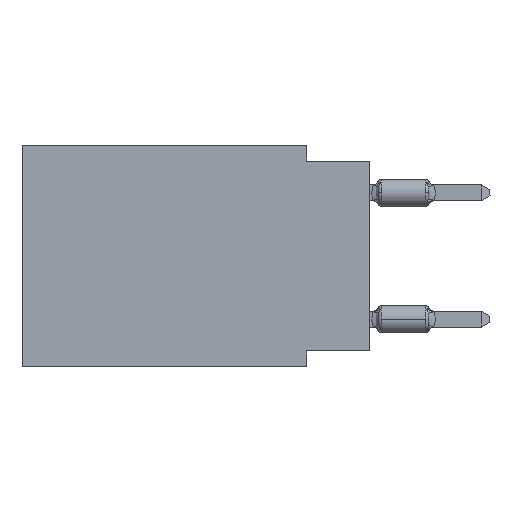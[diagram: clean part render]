
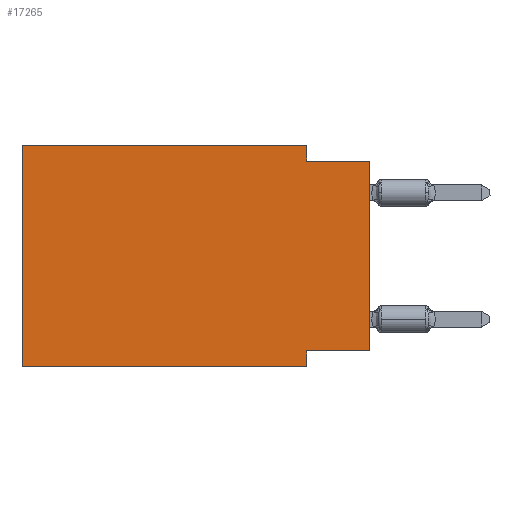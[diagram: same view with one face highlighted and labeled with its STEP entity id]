
A CAD part, left-side view. The second image highlights one B-rep face of the part: STEP entity #17265.
In plain terms, the highlighted planar face has unit normal (-1, 0, 0).
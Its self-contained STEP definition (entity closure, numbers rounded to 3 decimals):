
#519 = VERTEX_POINT ( 'NONE', #16517 ) ;
#940 = CARTESIAN_POINT ( 'NONE',  ( 0., 0., -0.635 ) ) ;
#1024 = LINE ( 'NONE', #8169, #1811 ) ;
#1096 = VERTEX_POINT ( 'NONE', #8989 ) ;
#1276 = VERTEX_POINT ( 'NONE', #13094 ) ;
#1332 = ORIENTED_EDGE ( 'NONE', *, *, #19990, .T. ) ;
#1726 = VERTEX_POINT ( 'NONE', #18130 ) ;
#1811 = VECTOR ( 'NONE', #10003, 1000. ) ;
#2099 = DIRECTION ( 'NONE',  ( 1., 0., 0. ) ) ;
#3362 = LINE ( 'NONE', #19885, #15245 ) ;
#3372 = ORIENTED_EDGE ( 'NONE', *, *, #19219, .F. ) ;
#3564 = ORIENTED_EDGE ( 'NONE', *, *, #18796, .F. ) ;
#4225 = CARTESIAN_POINT ( 'NONE',  ( 0., 0., 0. ) ) ;
#4650 = EDGE_CURVE ( 'NONE', #1726, #1096, #1024, .T. ) ;
#5056 = CARTESIAN_POINT ( 'NONE',  ( 0., 13.97, 0. ) ) ;
#5437 = DIRECTION ( 'NONE',  ( 0., 0., -1. ) ) ;
#5679 = VECTOR ( 'NONE', #12805, 1000. ) ;
#6331 = LINE ( 'NONE', #5056, #10864 ) ;
#6379 = VERTEX_POINT ( 'NONE', #21071 ) ;
#6448 = DIRECTION ( 'NONE',  ( 0., 1., 0. ) ) ;
#6913 = ORIENTED_EDGE ( 'NONE', *, *, #20837, .F. ) ;
#7190 = VECTOR ( 'NONE', #6448, 1000. ) ;
#7294 = PLANE ( 'NONE',  #21196 ) ;
#7486 = ORIENTED_EDGE ( 'NONE', *, *, #20045, .T. ) ;
#7638 = EDGE_CURVE ( 'NONE', #1096, #1276, #22091, .T. ) ;
#7876 = VECTOR ( 'NONE', #18262, 1000. ) ;
#8169 = CARTESIAN_POINT ( 'NONE',  ( 0., 2.54, 0. ) ) ;
#8708 = VERTEX_POINT ( 'NONE', #17564 ) ;
#8989 = CARTESIAN_POINT ( 'NONE',  ( 0., 2.54, -0.635 ) ) ;
#8993 = VECTOR ( 'NONE', #14712, 1000. ) ;
#9043 = ORIENTED_EDGE ( 'NONE', *, *, #12659, .F. ) ;
#9249 = FACE_OUTER_BOUND ( 'NONE', #22608, .T. ) ;
#9474 = LINE ( 'NONE', #19809, #5679 ) ;
#9628 = VECTOR ( 'NONE', #11522, 1000. ) ;
#10003 = DIRECTION ( 'NONE',  ( 0., 0., -1. ) ) ;
#10072 = ORIENTED_EDGE ( 'NONE', *, *, #4650, .F. ) ;
#10356 = DIRECTION ( 'NONE',  ( 0., 0., 1. ) ) ;
#10629 = CARTESIAN_POINT ( 'NONE',  ( 0., 13.97, -8.89 ) ) ;
#10864 = VECTOR ( 'NONE', #10356, 1000. ) ;
#11522 = DIRECTION ( 'NONE',  ( 0., -1., 0. ) ) ;
#12019 = CARTESIAN_POINT ( 'NONE',  ( 0., 13.97, -8.89 ) ) ;
#12659 = EDGE_CURVE ( 'NONE', #17247, #6379, #6331, .T. ) ;
#12805 = DIRECTION ( 'NONE',  ( 0., 0., -1. ) ) ;
#13094 = CARTESIAN_POINT ( 'NONE',  ( 0., 0., -0.635 ) ) ;
#13566 = ORIENTED_EDGE ( 'NONE', *, *, #7638, .F. ) ;
#14712 = DIRECTION ( 'NONE',  ( 0., -1., 0. ) ) ;
#14821 = LINE ( 'NONE', #12019, #8993 ) ;
#15198 = CARTESIAN_POINT ( 'NONE',  ( 0., 0., -8.255 ) ) ;
#15245 = VECTOR ( 'NONE', #21507, 1000. ) ;
#16517 = CARTESIAN_POINT ( 'NONE',  ( 0., 0., -8.255 ) ) ;
#17247 = VERTEX_POINT ( 'NONE', #10629 ) ;
#17265 = ADVANCED_FACE ( 'NONE', ( #9249 ), #7294, .F. ) ;
#17564 = CARTESIAN_POINT ( 'NONE',  ( 0., 2.54, -8.89 ) ) ;
#17629 = CARTESIAN_POINT ( 'NONE',  ( 0., 2.54, -8.255 ) ) ;
#17977 = CARTESIAN_POINT ( 'NONE',  ( 0., 13.97, 0. ) ) ;
#18130 = CARTESIAN_POINT ( 'NONE',  ( 0., 2.54, 0. ) ) ;
#18262 = DIRECTION ( 'NONE',  ( 0., 0., 1. ) ) ;
#18796 = EDGE_CURVE ( 'NONE', #20500, #8708, #9474, .T. ) ;
#19219 = EDGE_CURVE ( 'NONE', #6379, #1726, #3362, .T. ) ;
#19809 = CARTESIAN_POINT ( 'NONE',  ( 0., 2.54, -8.89 ) ) ;
#19885 = CARTESIAN_POINT ( 'NONE',  ( 0., 13.97, 0. ) ) ;
#19967 = LINE ( 'NONE', #4225, #7876 ) ;
#19990 = EDGE_CURVE ( 'NONE', #17247, #8708, #14821, .T. ) ;
#20045 = EDGE_CURVE ( 'NONE', #519, #1276, #19967, .T. ) ;
#20500 = VERTEX_POINT ( 'NONE', #17629 ) ;
#20837 = EDGE_CURVE ( 'NONE', #519, #20500, #22076, .T. ) ;
#21071 = CARTESIAN_POINT ( 'NONE',  ( 0., 13.97, 0. ) ) ;
#21196 = AXIS2_PLACEMENT_3D ( 'NONE', #17977, #2099, #5437 ) ;
#21507 = DIRECTION ( 'NONE',  ( 0., -1., 0. ) ) ;
#22076 = LINE ( 'NONE', #15198, #7190 ) ;
#22091 = LINE ( 'NONE', #940, #9628 ) ;
#22608 = EDGE_LOOP ( 'NONE', ( #7486, #13566, #10072, #3372, #9043, #1332, #3564, #6913 ) ) ;
